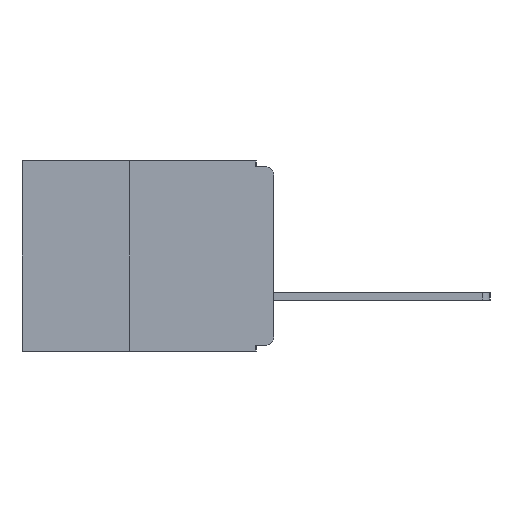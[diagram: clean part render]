
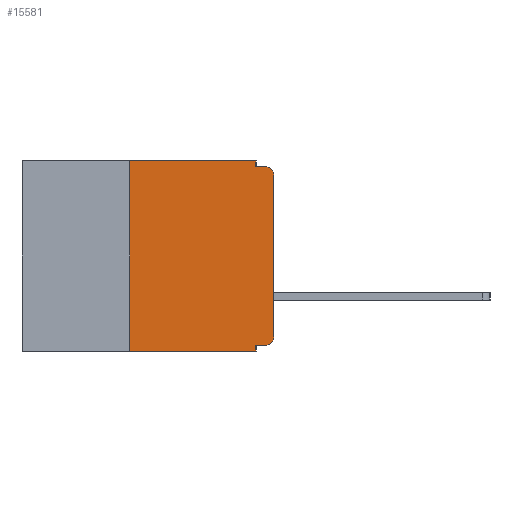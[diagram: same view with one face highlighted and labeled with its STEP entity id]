
A CAD part, left-side view. The second image highlights one B-rep face of the part: STEP entity #15581.
In plain terms, the highlighted planar face has unit normal (-1, 0, 0).
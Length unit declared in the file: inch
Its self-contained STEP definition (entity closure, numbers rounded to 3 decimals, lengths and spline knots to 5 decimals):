
#465 = VECTOR ( 'NONE', #9241, 39.37008 ) ;
#836 = VERTEX_POINT ( 'NONE', #6313 ) ;
#865 = VERTEX_POINT ( 'NONE', #12180 ) ;
#941 = VECTOR ( 'NONE', #13685, 39.37008 ) ;
#1048 = CARTESIAN_POINT ( 'NONE',  ( 0., 0., -0.025 ) ) ;
#1504 = CARTESIAN_POINT ( 'NONE',  ( 0., 0.031, -0.33 ) ) ;
#1631 = DIRECTION ( 'NONE',  ( 0., 0., -1. ) ) ;
#1886 = CARTESIAN_POINT ( 'NONE',  ( 0., 0.015, -0.305 ) ) ;
#2328 = VERTEX_POINT ( 'NONE', #13849 ) ;
#3319 = EDGE_CURVE ( 'NONE', #5629, #5977, #9289, .T. ) ;
#3470 = DIRECTION ( 'NONE',  ( 0., 0., -1. ) ) ;
#3751 = CARTESIAN_POINT ( 'NONE',  ( 0., 0.015, -0.32 ) ) ;
#3827 = VERTEX_POINT ( 'NONE', #3751 ) ;
#4232 = AXIS2_PLACEMENT_3D ( 'NONE', #15207, #5856, #16787 ) ;
#4412 = DIRECTION ( 'NONE',  ( 0., -1., 0. ) ) ;
#4415 = EDGE_CURVE ( 'NONE', #7823, #865, #12199, .T. ) ;
#4649 = LINE ( 'NONE', #18562, #465 ) ;
#5261 = EDGE_CURVE ( 'NONE', #14768, #7823, #12642, .T. ) ;
#5629 = VERTEX_POINT ( 'NONE', #6820 ) ;
#5856 = DIRECTION ( 'NONE',  ( -1., 0., 0. ) ) ;
#5977 = VERTEX_POINT ( 'NONE', #1048 ) ;
#6313 = CARTESIAN_POINT ( 'NONE',  ( 0., 0.031, -0.32 ) ) ;
#6820 = CARTESIAN_POINT ( 'NONE',  ( 0., 0., -0.305 ) ) ;
#7306 = DIRECTION ( 'NONE',  ( 1., 0., 0. ) ) ;
#7323 = ORIENTED_EDGE ( 'NONE', *, *, #3319, .T. ) ;
#7338 = LINE ( 'NONE', #17219, #11050 ) ;
#7484 = VECTOR ( 'NONE', #17272, 39.37008 ) ;
#7535 = EDGE_CURVE ( 'NONE', #9716, #2328, #10515, .T. ) ;
#7823 = VERTEX_POINT ( 'NONE', #8506 ) ;
#7952 = CIRCLE ( 'NONE', #4232, 0.015 ) ;
#8012 = VECTOR ( 'NONE', #16482, 39.37008 ) ;
#8101 = ORIENTED_EDGE ( 'NONE', *, *, #19592, .F. ) ;
#8141 = ORIENTED_EDGE ( 'NONE', *, *, #9723, .T. ) ;
#8506 = CARTESIAN_POINT ( 'NONE',  ( 0., 0.031, -0.01 ) ) ;
#9076 = CARTESIAN_POINT ( 'NONE',  ( 0., 0.437, -0.33 ) ) ;
#9241 = DIRECTION ( 'NONE',  ( 0., 1., 0. ) ) ;
#9289 = LINE ( 'NONE', #10473, #941 ) ;
#9331 = EDGE_CURVE ( 'NONE', #2328, #14768, #15783, .T. ) ;
#9716 = VERTEX_POINT ( 'NONE', #12044 ) ;
#9723 = EDGE_CURVE ( 'NONE', #5977, #865, #7952, .T. ) ;
#9775 = EDGE_CURVE ( 'NONE', #9716, #12450, #15270, .T. ) ;
#10018 = VECTOR ( 'NONE', #18737, 39.37008 ) ;
#10088 = AXIS2_PLACEMENT_3D ( 'NONE', #11988, #7306, #18212 ) ;
#10473 = CARTESIAN_POINT ( 'NONE',  ( 0., 0., 0. ) ) ;
#10515 = LINE ( 'NONE', #17185, #10018 ) ;
#10876 = ORIENTED_EDGE ( 'NONE', *, *, #7535, .F. ) ;
#11050 = VECTOR ( 'NONE', #1631, 39.37008 ) ;
#11246 = EDGE_LOOP ( 'NONE', ( #7323, #8141, #19485, #11612, #12605, #10876, #17991, #18018, #8101, #12977 ) ) ;
#11608 = CARTESIAN_POINT ( 'NONE',  ( 0., 0.031, 0. ) ) ;
#11612 = ORIENTED_EDGE ( 'NONE', *, *, #5261, .F. ) ;
#11988 = CARTESIAN_POINT ( 'NONE',  ( 0., 0.437, 0. ) ) ;
#12037 = CARTESIAN_POINT ( 'NONE',  ( 0., 0.031, 0. ) ) ;
#12044 = CARTESIAN_POINT ( 'NONE',  ( 0., 0.25, -0.33 ) ) ;
#12078 = DIRECTION ( 'NONE',  ( 0., 0., -1. ) ) ;
#12180 = CARTESIAN_POINT ( 'NONE',  ( 0., 0.015, -0.01 ) ) ;
#12199 = LINE ( 'NONE', #17248, #8012 ) ;
#12450 = VERTEX_POINT ( 'NONE', #1504 ) ;
#12605 = ORIENTED_EDGE ( 'NONE', *, *, #9331, .F. ) ;
#12642 = LINE ( 'NONE', #12037, #15787 ) ;
#12858 = DIRECTION ( 'NONE',  ( -1., 0., 0. ) ) ;
#12977 = ORIENTED_EDGE ( 'NONE', *, *, #19769, .T. ) ;
#13142 = AXIS2_PLACEMENT_3D ( 'NONE', #1886, #12858, #3470 ) ;
#13685 = DIRECTION ( 'NONE',  ( 0., 0., 1. ) ) ;
#13849 = CARTESIAN_POINT ( 'NONE',  ( 0., 0.25, 0. ) ) ;
#14768 = VERTEX_POINT ( 'NONE', #11608 ) ;
#14780 = VECTOR ( 'NONE', #4412, 39.37008 ) ;
#15207 = CARTESIAN_POINT ( 'NONE',  ( 0., 0.015, -0.025 ) ) ;
#15270 = LINE ( 'NONE', #9076, #14780 ) ;
#15581 = ADVANCED_FACE ( 'NONE', ( #19964 ), #16661, .F. ) ;
#15783 = LINE ( 'NONE', #18825, #7484 ) ;
#15787 = VECTOR ( 'NONE', #12078, 39.37008 ) ;
#16482 = DIRECTION ( 'NONE',  ( 0., -1., 0. ) ) ;
#16661 = PLANE ( 'NONE',  #10088 ) ;
#16787 = DIRECTION ( 'NONE',  ( 0., 0., -1. ) ) ;
#17185 = CARTESIAN_POINT ( 'NONE',  ( 0., 0.25, -0.33 ) ) ;
#17219 = CARTESIAN_POINT ( 'NONE',  ( 0., 0.031, -0.33 ) ) ;
#17248 = CARTESIAN_POINT ( 'NONE',  ( 0., 0., -0.01 ) ) ;
#17272 = DIRECTION ( 'NONE',  ( 0., -1., 0. ) ) ;
#17820 = CIRCLE ( 'NONE', #13142, 0.015 ) ;
#17991 = ORIENTED_EDGE ( 'NONE', *, *, #9775, .T. ) ;
#18018 = ORIENTED_EDGE ( 'NONE', *, *, #19685, .F. ) ;
#18212 = DIRECTION ( 'NONE',  ( 0., 0., -1. ) ) ;
#18562 = CARTESIAN_POINT ( 'NONE',  ( 0., 0., -0.32 ) ) ;
#18737 = DIRECTION ( 'NONE',  ( 0., 0., 1. ) ) ;
#18825 = CARTESIAN_POINT ( 'NONE',  ( 0., 0.437, 0. ) ) ;
#19485 = ORIENTED_EDGE ( 'NONE', *, *, #4415, .F. ) ;
#19592 = EDGE_CURVE ( 'NONE', #3827, #836, #4649, .T. ) ;
#19685 = EDGE_CURVE ( 'NONE', #836, #12450, #7338, .T. ) ;
#19769 = EDGE_CURVE ( 'NONE', #3827, #5629, #17820, .T. ) ;
#19964 = FACE_OUTER_BOUND ( 'NONE', #11246, .T. ) ;
